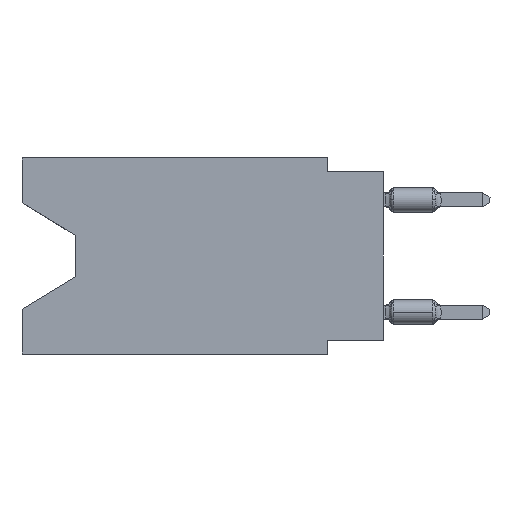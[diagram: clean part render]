
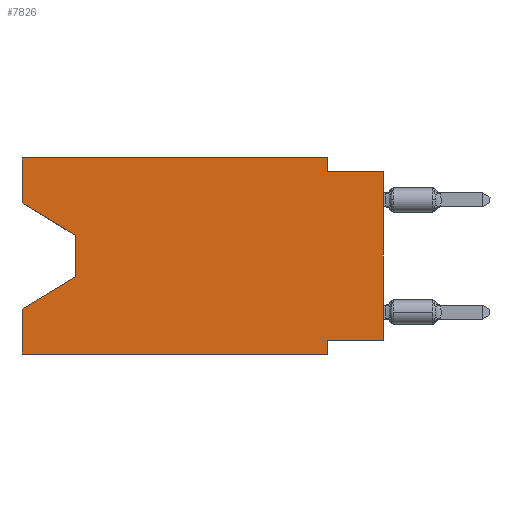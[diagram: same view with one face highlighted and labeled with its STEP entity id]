
A CAD part, left-side view. The second image highlights one B-rep face of the part: STEP entity #7826.
In plain terms, the highlighted planar face has unit normal (-1, 0, 0).
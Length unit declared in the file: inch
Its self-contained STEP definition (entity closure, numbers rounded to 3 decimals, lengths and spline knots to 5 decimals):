
#49 = VECTOR ( 'NONE', #12479, 39.37008 ) ;
#72 = VECTOR ( 'NONE', #3146, 39.37008 ) ;
#77 = VERTEX_POINT ( 'NONE', #10882 ) ;
#144 = EDGE_CURVE ( 'NONE', #10938, #6118, #3914, .T. ) ;
#507 = DIRECTION ( 'NONE',  ( 0., 0., -1. ) ) ;
#515 = VECTOR ( 'NONE', #5586, 39.37008 ) ;
#791 = CARTESIAN_POINT ( 'NONE',  ( 0., 0.1, -0.325 ) ) ;
#851 = VECTOR ( 'NONE', #15537, 39.37008 ) ;
#1199 = ORIENTED_EDGE ( 'NONE', *, *, #7296, .F. ) ;
#1221 = EDGE_CURVE ( 'NONE', #13034, #15154, #14714, .T. ) ;
#2203 = ORIENTED_EDGE ( 'NONE', *, *, #17872, .T. ) ;
#2393 = CARTESIAN_POINT ( 'NONE',  ( 0., 0.645, 0. ) ) ;
#2897 = VERTEX_POINT ( 'NONE', #5958 ) ;
#3000 = CARTESIAN_POINT ( 'NONE',  ( 0., 0.55, -0.212 ) ) ;
#3146 = DIRECTION ( 'NONE',  ( 0., 0., 1. ) ) ;
#3230 = EDGE_CURVE ( 'NONE', #2897, #11799, #12650, .T. ) ;
#3861 = DIRECTION ( 'NONE',  ( 0., 1., 0. ) ) ;
#3914 = LINE ( 'NONE', #16550, #515 ) ;
#4126 = ORIENTED_EDGE ( 'NONE', *, *, #7701, .F. ) ;
#4145 = CARTESIAN_POINT ( 'NONE',  ( 0., 0.645, 0. ) ) ;
#4192 = CARTESIAN_POINT ( 'NONE',  ( 0., 0., -0.025 ) ) ;
#4554 = CARTESIAN_POINT ( 'NONE',  ( 0., 0., 0. ) ) ;
#4605 = EDGE_LOOP ( 'NONE', ( #16311, #6922, #8619, #1199, #7081, #7500, #4126, #2203, #9608, #17547, #14190, #5657 ) ) ;
#4926 = CARTESIAN_POINT ( 'NONE',  ( 0., 0.55, -0.212 ) ) ;
#4985 = CARTESIAN_POINT ( 'NONE',  ( 0., 0.645, 0. ) ) ;
#5154 = CARTESIAN_POINT ( 'NONE',  ( 0., 0.1, 0. ) ) ;
#5197 = LINE ( 'NONE', #2393, #7024 ) ;
#5323 = VERTEX_POINT ( 'NONE', #5668 ) ;
#5358 = DIRECTION ( 'NONE',  ( 0., -1., 0. ) ) ;
#5546 = VECTOR ( 'NONE', #3861, 39.37008 ) ;
#5586 = DIRECTION ( 'NONE',  ( 0., 0., -1. ) ) ;
#5598 = VECTOR ( 'NONE', #14978, 39.37008 ) ;
#5657 = ORIENTED_EDGE ( 'NONE', *, *, #16638, .F. ) ;
#5668 = CARTESIAN_POINT ( 'NONE',  ( 0., 0.55, -0.138 ) ) ;
#5848 = CARTESIAN_POINT ( 'NONE',  ( 0., 0.645, -0.08025 ) ) ;
#5958 = CARTESIAN_POINT ( 'NONE',  ( 0., 0.1, -0.025 ) ) ;
#5985 = CARTESIAN_POINT ( 'NONE',  ( 0., 0.1, 0. ) ) ;
#6118 = VERTEX_POINT ( 'NONE', #15910 ) ;
#6275 = VECTOR ( 'NONE', #5358, 39.37008 ) ;
#6732 = DIRECTION ( 'NONE',  ( 0., 0., 1. ) ) ;
#6922 = ORIENTED_EDGE ( 'NONE', *, *, #14847, .T. ) ;
#6956 = LINE ( 'NONE', #16460, #5598 ) ;
#7024 = VECTOR ( 'NONE', #8160, 39.37008 ) ;
#7081 = ORIENTED_EDGE ( 'NONE', *, *, #16202, .T. ) ;
#7274 = VERTEX_POINT ( 'NONE', #9822 ) ;
#7296 = EDGE_CURVE ( 'NONE', #7274, #15154, #5197, .T. ) ;
#7393 = LINE ( 'NONE', #10559, #16130 ) ;
#7500 = ORIENTED_EDGE ( 'NONE', *, *, #144, .F. ) ;
#7662 = VECTOR ( 'NONE', #8669, 39.37008 ) ;
#7701 = EDGE_CURVE ( 'NONE', #77, #10938, #17984, .T. ) ;
#7718 = VERTEX_POINT ( 'NONE', #4145 ) ;
#7826 = ADVANCED_FACE ( 'NONE', ( #15568 ), #12686, .F. ) ;
#8160 = DIRECTION ( 'NONE',  ( 0., 0., 1. ) ) ;
#8619 = ORIENTED_EDGE ( 'NONE', *, *, #1221, .T. ) ;
#8669 = DIRECTION ( 'NONE',  ( 0., 0.855, -0.519 ) ) ;
#8722 = VERTEX_POINT ( 'NONE', #5154 ) ;
#9344 = EDGE_CURVE ( 'NONE', #12908, #5323, #6956, .T. ) ;
#9608 = ORIENTED_EDGE ( 'NONE', *, *, #3230, .F. ) ;
#9822 = CARTESIAN_POINT ( 'NONE',  ( 0., 0.645, -0.35 ) ) ;
#9935 = LINE ( 'NONE', #4554, #72 ) ;
#10559 = CARTESIAN_POINT ( 'NONE',  ( 0., 0.55, -0.138 ) ) ;
#10657 = EDGE_CURVE ( 'NONE', #8722, #2897, #13229, .T. ) ;
#10882 = CARTESIAN_POINT ( 'NONE',  ( 0., 0., -0.325 ) ) ;
#10938 = VERTEX_POINT ( 'NONE', #791 ) ;
#11366 = VECTOR ( 'NONE', #14722, 39.37008 ) ;
#11613 = VECTOR ( 'NONE', #6732, 39.37008 ) ;
#11799 = VERTEX_POINT ( 'NONE', #14964 ) ;
#12227 = CARTESIAN_POINT ( 'NONE',  ( 0., 0., -0.325 ) ) ;
#12388 = AXIS2_PLACEMENT_3D ( 'NONE', #14436, #18362, #17230 ) ;
#12479 = DIRECTION ( 'NONE',  ( 0., -1., 0. ) ) ;
#12650 = LINE ( 'NONE', #4192, #851 ) ;
#12686 = PLANE ( 'NONE',  #12388 ) ;
#12908 = VERTEX_POINT ( 'NONE', #5848 ) ;
#13034 = VERTEX_POINT ( 'NONE', #4926 ) ;
#13229 = LINE ( 'NONE', #5985, #11366 ) ;
#14190 = ORIENTED_EDGE ( 'NONE', *, *, #17313, .F. ) ;
#14436 = CARTESIAN_POINT ( 'NONE',  ( 0., 0.645, 0. ) ) ;
#14714 = LINE ( 'NONE', #3000, #7662 ) ;
#14722 = DIRECTION ( 'NONE',  ( 0., 0., -1. ) ) ;
#14847 = EDGE_CURVE ( 'NONE', #5323, #13034, #7393, .T. ) ;
#14964 = CARTESIAN_POINT ( 'NONE',  ( 0., 0., -0.025 ) ) ;
#14978 = DIRECTION ( 'NONE',  ( 0., -0.855, -0.519 ) ) ;
#15154 = VERTEX_POINT ( 'NONE', #18361 ) ;
#15352 = CARTESIAN_POINT ( 'NONE',  ( 0., 0.645, 0. ) ) ;
#15537 = DIRECTION ( 'NONE',  ( 0., -1., 0. ) ) ;
#15568 = FACE_OUTER_BOUND ( 'NONE', #4605, .T. ) ;
#15910 = CARTESIAN_POINT ( 'NONE',  ( 0., 0.1, -0.35 ) ) ;
#16130 = VECTOR ( 'NONE', #507, 39.37008 ) ;
#16202 = EDGE_CURVE ( 'NONE', #7274, #6118, #16420, .T. ) ;
#16311 = ORIENTED_EDGE ( 'NONE', *, *, #9344, .T. ) ;
#16420 = LINE ( 'NONE', #18090, #6275 ) ;
#16460 = CARTESIAN_POINT ( 'NONE',  ( 0., 0.645, -0.08025 ) ) ;
#16487 = LINE ( 'NONE', #4985, #11613 ) ;
#16550 = CARTESIAN_POINT ( 'NONE',  ( 0., 0.1, -0.35 ) ) ;
#16638 = EDGE_CURVE ( 'NONE', #12908, #7718, #16487, .T. ) ;
#17230 = DIRECTION ( 'NONE',  ( 0., 0., -1. ) ) ;
#17313 = EDGE_CURVE ( 'NONE', #7718, #8722, #18329, .T. ) ;
#17547 = ORIENTED_EDGE ( 'NONE', *, *, #10657, .F. ) ;
#17872 = EDGE_CURVE ( 'NONE', #77, #11799, #9935, .T. ) ;
#17984 = LINE ( 'NONE', #12227, #5546 ) ;
#18090 = CARTESIAN_POINT ( 'NONE',  ( 0., 0.645, -0.35 ) ) ;
#18329 = LINE ( 'NONE', #15352, #49 ) ;
#18361 = CARTESIAN_POINT ( 'NONE',  ( 0., 0.645, -0.26975 ) ) ;
#18362 = DIRECTION ( 'NONE',  ( 1., 0., 0. ) ) ;
